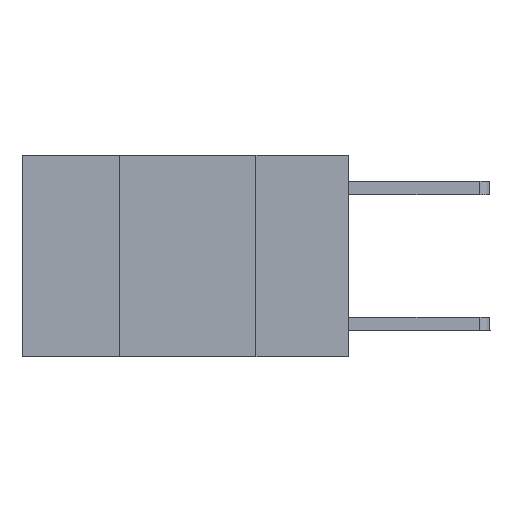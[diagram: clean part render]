
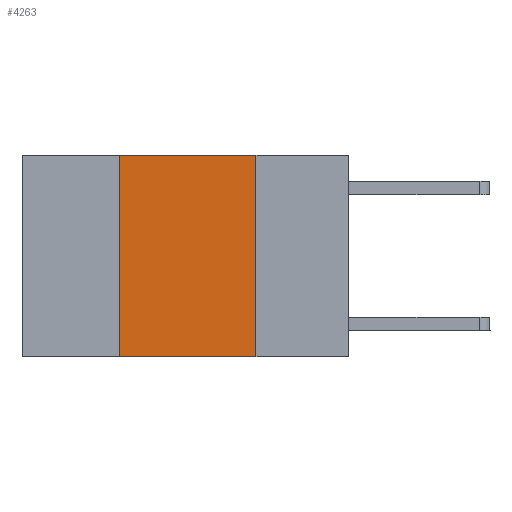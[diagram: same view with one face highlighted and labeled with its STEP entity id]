
A CAD part, left-side view. The second image highlights one B-rep face of the part: STEP entity #4263.
In plain terms, the highlighted planar face has unit normal (-1, 0, 0).
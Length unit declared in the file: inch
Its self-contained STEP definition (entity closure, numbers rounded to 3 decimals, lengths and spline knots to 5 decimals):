
#71 = VECTOR ( 'NONE', #7821, 39.37008 ) ;
#338 = DIRECTION ( 'NONE',  ( 0., -1., 0. ) ) ;
#419 = LINE ( 'NONE', #4357, #8305 ) ;
#1370 = DIRECTION ( 'NONE',  ( 1., 0., 0. ) ) ;
#1431 = EDGE_LOOP ( 'NONE', ( #4602, #6555, #8795, #5319 ) ) ;
#1648 = EDGE_CURVE ( 'NONE', #5902, #6878, #419, .T. ) ;
#1858 = EDGE_CURVE ( 'NONE', #6878, #5800, #9481, .T. ) ;
#1989 = EDGE_CURVE ( 'NONE', #8514, #5902, #4093, .T. ) ;
#2045 = VECTOR ( 'NONE', #338, 39.37008 ) ;
#2226 = CARTESIAN_POINT ( 'NONE',  ( 0., 0.42, 0. ) ) ;
#2314 = LINE ( 'NONE', #8671, #2045 ) ;
#2999 = FACE_OUTER_BOUND ( 'NONE', #1431, .T. ) ;
#3137 = CARTESIAN_POINT ( 'NONE',  ( 0., 0.42, 0. ) ) ;
#3395 = VECTOR ( 'NONE', #9520, 39.37008 ) ;
#3711 = DIRECTION ( 'NONE',  ( 0., -1., 0. ) ) ;
#4093 = LINE ( 'NONE', #3137, #71 ) ;
#4184 = CARTESIAN_POINT ( 'NONE',  ( 0., 0.17, 0. ) ) ;
#4263 = ADVANCED_FACE ( 'NONE', ( #2999 ), #8220, .F. ) ;
#4357 = CARTESIAN_POINT ( 'NONE',  ( 0., 0.6, 0. ) ) ;
#4602 = ORIENTED_EDGE ( 'NONE', *, *, #1858, .F. ) ;
#5319 = ORIENTED_EDGE ( 'NONE', *, *, #5539, .T. ) ;
#5539 = EDGE_CURVE ( 'NONE', #8514, #5800, #2314, .T. ) ;
#5800 = VERTEX_POINT ( 'NONE', #6828 ) ;
#5902 = VERTEX_POINT ( 'NONE', #2226 ) ;
#6167 = CARTESIAN_POINT ( 'NONE',  ( 0., 0.6, 0. ) ) ;
#6555 = ORIENTED_EDGE ( 'NONE', *, *, #1648, .F. ) ;
#6828 = CARTESIAN_POINT ( 'NONE',  ( 0., 0.17, -0.37 ) ) ;
#6854 = DIRECTION ( 'NONE',  ( 0., 0., -1. ) ) ;
#6878 = VERTEX_POINT ( 'NONE', #4184 ) ;
#7821 = DIRECTION ( 'NONE',  ( 0., 0., 1. ) ) ;
#7879 = CARTESIAN_POINT ( 'NONE',  ( 0., 0.17, 0. ) ) ;
#7954 = AXIS2_PLACEMENT_3D ( 'NONE', #6167, #1370, #6854 ) ;
#8220 = PLANE ( 'NONE',  #7954 ) ;
#8305 = VECTOR ( 'NONE', #3711, 39.37008 ) ;
#8514 = VERTEX_POINT ( 'NONE', #9561 ) ;
#8671 = CARTESIAN_POINT ( 'NONE',  ( 0., 0.6, -0.37 ) ) ;
#8795 = ORIENTED_EDGE ( 'NONE', *, *, #1989, .F. ) ;
#9481 = LINE ( 'NONE', #7879, #3395 ) ;
#9520 = DIRECTION ( 'NONE',  ( 0., 0., -1. ) ) ;
#9561 = CARTESIAN_POINT ( 'NONE',  ( 0., 0.42, -0.37 ) ) ;
